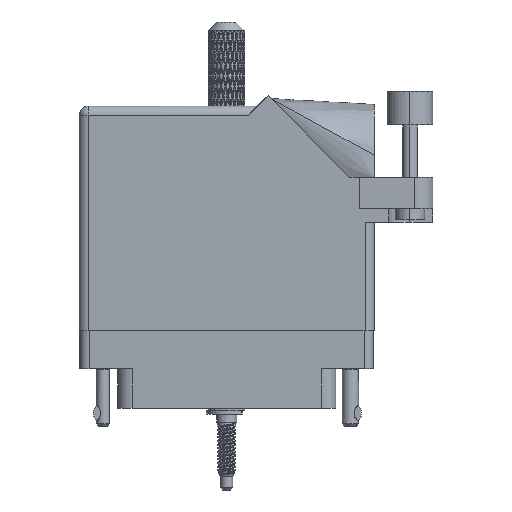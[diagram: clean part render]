
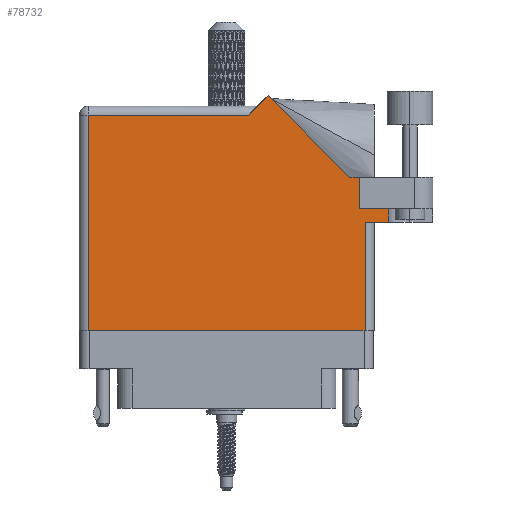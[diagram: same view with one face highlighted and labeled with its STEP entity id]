
A CAD part, front view. The second image highlights one B-rep face of the part: STEP entity #78732.
In plain terms, the highlighted face is planar.
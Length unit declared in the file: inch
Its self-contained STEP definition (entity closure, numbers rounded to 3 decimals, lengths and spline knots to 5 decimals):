
#402 = CARTESIAN_POINT ( 'NONE',  ( 1.948, 0.737, 0. ) ) ;
#1464 = LINE ( 'NONE', #31868, #63400 ) ;
#3329 = LINE ( 'NONE', #71969, #23994 ) ;
#3855 = CARTESIAN_POINT ( 'NONE',  ( 1.91, 0.831, 0. ) ) ;
#4192 = LINE ( 'NONE', #15453, #75796 ) ;
#4292 = CARTESIAN_POINT ( 'NONE',  ( 1.155, 1.468, 0. ) ) ;
#5571 = PLANE ( 'NONE',  #76564 ) ;
#9882 = DIRECTION ( 'NONE',  ( -0.707, -0.707, 0. ) ) ;
#10981 = EDGE_CURVE ( 'NONE', #11050, #55167, #47728, .T. ) ;
#11050 = VERTEX_POINT ( 'NONE', #28436 ) ;
#13456 = ORIENTED_EDGE ( 'NONE', *, *, #49331, .T. ) ;
#14910 = VERTEX_POINT ( 'NONE', #4292 ) ;
#15453 = CARTESIAN_POINT ( 'NONE',  ( 2.01, 0.737, 0. ) ) ;
#18391 = CARTESIAN_POINT ( 'NONE',  ( 1.91, 1.044, 0. ) ) ;
#19360 = LINE ( 'NONE', #33084, #63415 ) ;
#19661 = EDGE_CURVE ( 'NONE', #21839, #41418, #30202, .T. ) ;
#21839 = VERTEX_POINT ( 'NONE', #52110 ) ;
#22180 = EDGE_CURVE ( 'NONE', #14910, #11050, #51408, .T. ) ;
#22385 = ORIENTED_EDGE ( 'NONE', *, *, #29106, .T. ) ;
#23418 = DIRECTION ( 'NONE',  ( 0., 1., 0. ) ) ;
#23994 = VECTOR ( 'NONE', #63083, 39.37008 ) ;
#24482 = EDGE_CURVE ( 'NONE', #41418, #49521, #19360, .T. ) ;
#26064 = ORIENTED_EDGE ( 'NONE', *, *, #24482, .F. ) ;
#26852 = EDGE_LOOP ( 'NONE', ( #22385, #89521, #72083, #26064, #107794, #75712, #56225, #13456, #104900, #75914, #68980 ) ) ;
#27521 = EDGE_CURVE ( 'NONE', #21839, #80140, #103238, .T. ) ;
#28436 = CARTESIAN_POINT ( 'NONE',  ( 0.062, 1.468, 0. ) ) ;
#29106 = EDGE_CURVE ( 'NONE', #55167, #55578, #62902, .T. ) ;
#29874 = CARTESIAN_POINT ( 'NONE',  ( 1.91, 0.831, 0. ) ) ;
#30202 = LINE ( 'NONE', #3855, #90955 ) ;
#31868 = CARTESIAN_POINT ( 'NONE',  ( 1.948, 0.737, 0. ) ) ;
#33084 = CARTESIAN_POINT ( 'NONE',  ( 2.1115, 1.16177, 0. ) ) ;
#34826 = VECTOR ( 'NONE', #9882, 39.37008 ) ;
#37560 = VECTOR ( 'NONE', #98972, 39.37008 ) ;
#41323 = DIRECTION ( 'NONE',  ( 0., 0., -1. ) ) ;
#41418 = VERTEX_POINT ( 'NONE', #77818 ) ;
#42772 = DIRECTION ( 'NONE',  ( 1., 0., 0. ) ) ;
#45778 = VERTEX_POINT ( 'NONE', #402 ) ;
#46022 = CARTESIAN_POINT ( 'NONE',  ( 1.948, 0., 0. ) ) ;
#47728 = LINE ( 'NONE', #89009, #114255 ) ;
#47870 = VERTEX_POINT ( 'NONE', #90682 ) ;
#49331 = EDGE_CURVE ( 'NONE', #47870, #74667, #56953, .T. ) ;
#49521 = VERTEX_POINT ( 'NONE', #92805 ) ;
#50695 = CARTESIAN_POINT ( 'NONE',  ( 1.28771, 1.60071, 0. ) ) ;
#51408 = LINE ( 'NONE', #88178, #37560 ) ;
#52110 = CARTESIAN_POINT ( 'NONE',  ( 1.91, 0.831, 0. ) ) ;
#55045 = EDGE_CURVE ( 'NONE', #80140, #47870, #3329, .T. ) ;
#55167 = VERTEX_POINT ( 'NONE', #109409 ) ;
#55578 = VERTEX_POINT ( 'NONE', #46022 ) ;
#56225 = ORIENTED_EDGE ( 'NONE', *, *, #55045, .T. ) ;
#56459 = EDGE_CURVE ( 'NONE', #74667, #14910, #88583, .T. ) ;
#56953 = LINE ( 'NONE', #102608, #95658 ) ;
#57359 = DIRECTION ( 'NONE',  ( 1., 0., 0. ) ) ;
#61216 = DIRECTION ( 'NONE',  ( 1., 0., 0. ) ) ;
#62902 = LINE ( 'NONE', #78558, #96096 ) ;
#63083 = DIRECTION ( 'NONE',  ( -1., 0., 0. ) ) ;
#63400 = VECTOR ( 'NONE', #23418, 39.37008 ) ;
#63415 = VECTOR ( 'NONE', #103652, 39.37008 ) ;
#64308 = FACE_OUTER_BOUND ( 'NONE', #26852, .T. ) ;
#67172 = CARTESIAN_POINT ( 'NONE',  ( 0., 1.53, 0. ) ) ;
#67692 = EDGE_CURVE ( 'NONE', #55578, #45778, #1464, .T. ) ;
#68980 = ORIENTED_EDGE ( 'NONE', *, *, #10981, .T. ) ;
#71969 = CARTESIAN_POINT ( 'NONE',  ( 2.41, 1.044, 0. ) ) ;
#72083 = ORIENTED_EDGE ( 'NONE', *, *, #110706, .T. ) ;
#74667 = VERTEX_POINT ( 'NONE', #50695 ) ;
#75611 = DIRECTION ( 'NONE',  ( -1., 0., 0. ) ) ;
#75712 = ORIENTED_EDGE ( 'NONE', *, *, #27521, .T. ) ;
#75796 = VECTOR ( 'NONE', #42772, 39.37008 ) ;
#75914 = ORIENTED_EDGE ( 'NONE', *, *, #22180, .T. ) ;
#76564 = AXIS2_PLACEMENT_3D ( 'NONE', #67172, #41323, #75611 ) ;
#77818 = CARTESIAN_POINT ( 'NONE',  ( 2.1115, 0.831, 0. ) ) ;
#78558 = CARTESIAN_POINT ( 'NONE',  ( 0., 0., 0. ) ) ;
#78732 = ADVANCED_FACE ( 'NONE', ( #64308 ), #5571, .F. ) ;
#80140 = VERTEX_POINT ( 'NONE', #18391 ) ;
#82661 = DIRECTION ( 'NONE',  ( 0., 1., 0. ) ) ;
#88178 = CARTESIAN_POINT ( 'NONE',  ( 0., 1.468, 0. ) ) ;
#88583 = LINE ( 'NONE', #107384, #34826 ) ;
#89009 = CARTESIAN_POINT ( 'NONE',  ( 0.062, 0., 0. ) ) ;
#89521 = ORIENTED_EDGE ( 'NONE', *, *, #67692, .T. ) ;
#90682 = CARTESIAN_POINT ( 'NONE',  ( 1.84442, 1.044, 0. ) ) ;
#90955 = VECTOR ( 'NONE', #57359, 39.37008 ) ;
#92805 = CARTESIAN_POINT ( 'NONE',  ( 2.1115, 0.737, 0. ) ) ;
#95658 = VECTOR ( 'NONE', #110754, 39.37008 ) ;
#96096 = VECTOR ( 'NONE', #61216, 39.37008 ) ;
#98972 = DIRECTION ( 'NONE',  ( -1., 0., 0. ) ) ;
#102608 = CARTESIAN_POINT ( 'NONE',  ( 1.84442, 1.044, 0. ) ) ;
#103238 = LINE ( 'NONE', #29874, #107330 ) ;
#103652 = DIRECTION ( 'NONE',  ( 0., -1., 0. ) ) ;
#104900 = ORIENTED_EDGE ( 'NONE', *, *, #56459, .T. ) ;
#106368 = DIRECTION ( 'NONE',  ( 0., -1., 0. ) ) ;
#107330 = VECTOR ( 'NONE', #82661, 39.37008 ) ;
#107384 = CARTESIAN_POINT ( 'NONE',  ( 1.217, 1.53, 0. ) ) ;
#107794 = ORIENTED_EDGE ( 'NONE', *, *, #19661, .F. ) ;
#109409 = CARTESIAN_POINT ( 'NONE',  ( 0.062, 0., 0. ) ) ;
#110706 = EDGE_CURVE ( 'NONE', #45778, #49521, #4192, .T. ) ;
#110754 = DIRECTION ( 'NONE',  ( -0.707, 0.707, 0. ) ) ;
#114255 = VECTOR ( 'NONE', #106368, 39.37008 ) ;
